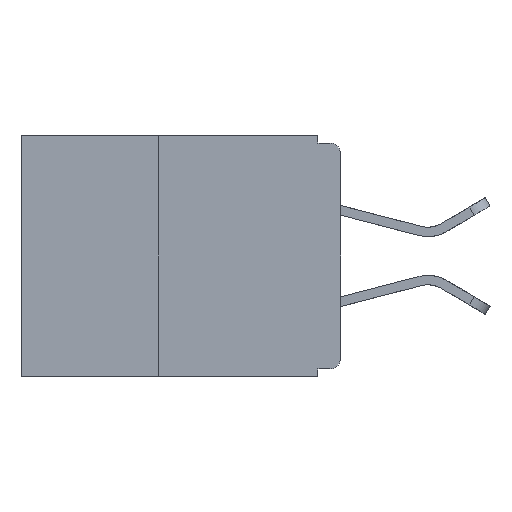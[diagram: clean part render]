
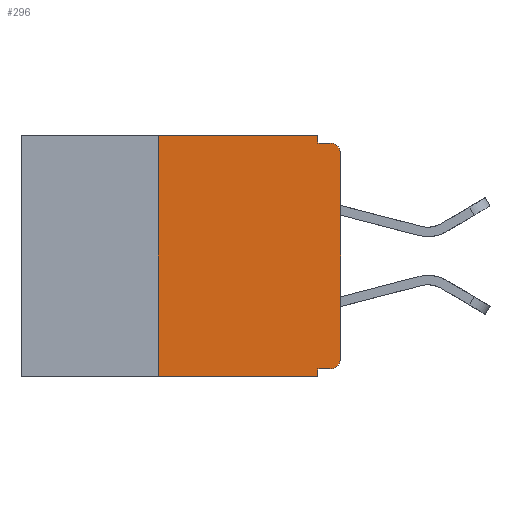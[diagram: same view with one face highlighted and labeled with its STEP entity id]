
A CAD part, left-side view. The second image highlights one B-rep face of the part: STEP entity #296.
In plain terms, the highlighted planar face has unit normal (-1, 0, 0).
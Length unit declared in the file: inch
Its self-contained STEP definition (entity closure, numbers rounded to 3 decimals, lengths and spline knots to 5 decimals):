
#296 = ADVANCED_FACE ( 'NONE', ( #11263 ), #28574, .F. ) ;
#948 = EDGE_CURVE ( 'NONE', #23775, #23313, #18565, .T. ) ;
#1109 = VERTEX_POINT ( 'NONE', #7180 ) ;
#1110 = EDGE_CURVE ( 'NONE', #29141, #15343, #18947, .T. ) ;
#1791 = CARTESIAN_POINT ( 'NONE',  ( 0., 0.25, -0.33 ) ) ;
#2021 = LINE ( 'NONE', #1791, #21980 ) ;
#2103 = CARTESIAN_POINT ( 'NONE',  ( 0., 0.031, 0. ) ) ;
#2149 = EDGE_LOOP ( 'NONE', ( #12521, #8941, #10522, #13044, #33105, #18104, #19551, #28504, #15742, #12851 ) ) ;
#2371 = VECTOR ( 'NONE', #25458, 39.37008 ) ;
#2438 = DIRECTION ( 'NONE',  ( 0., 0., -1. ) ) ;
#3979 = DIRECTION ( 'NONE',  ( 0., 0., 1. ) ) ;
#4432 = DIRECTION ( 'NONE',  ( 0., 0., 1. ) ) ;
#4693 = CARTESIAN_POINT ( 'NONE',  ( 0., 0.015, -0.01 ) ) ;
#4738 = CARTESIAN_POINT ( 'NONE',  ( 0., 0.437, 0. ) ) ;
#5278 = AXIS2_PLACEMENT_3D ( 'NONE', #27246, #6772, #20727 ) ;
#6495 = LINE ( 'NONE', #17017, #11788 ) ;
#6772 = DIRECTION ( 'NONE',  ( 1., 0., 0. ) ) ;
#7180 = CARTESIAN_POINT ( 'NONE',  ( 0., 0., -0.025 ) ) ;
#7373 = DIRECTION ( 'NONE',  ( 0., -1., 0. ) ) ;
#7431 = DIRECTION ( 'NONE',  ( -1., 0., 0. ) ) ;
#7521 = CIRCLE ( 'NONE', #15760, 0.015 ) ;
#8125 = DIRECTION ( 'NONE',  ( -1., 0., 0. ) ) ;
#8941 = ORIENTED_EDGE ( 'NONE', *, *, #21739, .T. ) ;
#10522 = ORIENTED_EDGE ( 'NONE', *, *, #11545, .F. ) ;
#11263 = FACE_OUTER_BOUND ( 'NONE', #2149, .T. ) ;
#11545 = EDGE_CURVE ( 'NONE', #23313, #26784, #32748, .T. ) ;
#11788 = VECTOR ( 'NONE', #3979, 39.37008 ) ;
#11990 = VECTOR ( 'NONE', #23617, 39.37008 ) ;
#12247 = VERTEX_POINT ( 'NONE', #26796 ) ;
#12361 = EDGE_CURVE ( 'NONE', #12247, #29141, #24601, .T. ) ;
#12521 = ORIENTED_EDGE ( 'NONE', *, *, #28033, .T. ) ;
#12851 = ORIENTED_EDGE ( 'NONE', *, *, #24973, .T. ) ;
#13044 = ORIENTED_EDGE ( 'NONE', *, *, #948, .F. ) ;
#13292 = EDGE_CURVE ( 'NONE', #14085, #23775, #30454, .T. ) ;
#13724 = CARTESIAN_POINT ( 'NONE',  ( 0., 0.031, -0.32 ) ) ;
#14085 = VERTEX_POINT ( 'NONE', #20985 ) ;
#15007 = VERTEX_POINT ( 'NONE', #32631 ) ;
#15147 = CARTESIAN_POINT ( 'NONE',  ( 0., 0.437, -0.33 ) ) ;
#15343 = VERTEX_POINT ( 'NONE', #16211 ) ;
#15742 = ORIENTED_EDGE ( 'NONE', *, *, #12361, .F. ) ;
#15760 = AXIS2_PLACEMENT_3D ( 'NONE', #23665, #8125, #26226 ) ;
#15841 = CARTESIAN_POINT ( 'NONE',  ( 0., 0.031, -0.33 ) ) ;
#16211 = CARTESIAN_POINT ( 'NONE',  ( 0., 0.031, -0.33 ) ) ;
#16932 = VECTOR ( 'NONE', #7373, 39.37008 ) ;
#17017 = CARTESIAN_POINT ( 'NONE',  ( 0., 0., 0. ) ) ;
#18104 = ORIENTED_EDGE ( 'NONE', *, *, #28184, .F. ) ;
#18565 = LINE ( 'NONE', #2103, #24544 ) ;
#18947 = LINE ( 'NONE', #15841, #11990 ) ;
#19045 = VERTEX_POINT ( 'NONE', #31705 ) ;
#19551 = ORIENTED_EDGE ( 'NONE', *, *, #28864, .T. ) ;
#20727 = DIRECTION ( 'NONE',  ( 0., 0., -1. ) ) ;
#20985 = CARTESIAN_POINT ( 'NONE',  ( 0., 0.25, 0. ) ) ;
#21359 = CIRCLE ( 'NONE', #27033, 0.015 ) ;
#21739 = EDGE_CURVE ( 'NONE', #1109, #26784, #7521, .T. ) ;
#21980 = VECTOR ( 'NONE', #4432, 39.37008 ) ;
#22987 = CARTESIAN_POINT ( 'NONE',  ( 0., 0.015, -0.305 ) ) ;
#23313 = VERTEX_POINT ( 'NONE', #30224 ) ;
#23617 = DIRECTION ( 'NONE',  ( 0., 0., -1. ) ) ;
#23665 = CARTESIAN_POINT ( 'NONE',  ( 0., 0.015, -0.025 ) ) ;
#23775 = VERTEX_POINT ( 'NONE', #31923 ) ;
#24544 = VECTOR ( 'NONE', #2438, 39.37008 ) ;
#24601 = LINE ( 'NONE', #32136, #29743 ) ;
#24973 = EDGE_CURVE ( 'NONE', #12247, #19045, #21359, .T. ) ;
#25299 = VECTOR ( 'NONE', #28945, 39.37008 ) ;
#25458 = DIRECTION ( 'NONE',  ( 0., -1., 0. ) ) ;
#25539 = DIRECTION ( 'NONE',  ( 0., 0., -1. ) ) ;
#26226 = DIRECTION ( 'NONE',  ( 0., 0., -1. ) ) ;
#26390 = CARTESIAN_POINT ( 'NONE',  ( 0., 0., -0.01 ) ) ;
#26784 = VERTEX_POINT ( 'NONE', #4693 ) ;
#26796 = CARTESIAN_POINT ( 'NONE',  ( 0., 0.015, -0.32 ) ) ;
#27033 = AXIS2_PLACEMENT_3D ( 'NONE', #22987, #7431, #25539 ) ;
#27246 = CARTESIAN_POINT ( 'NONE',  ( 0., 0.437, 0. ) ) ;
#28033 = EDGE_CURVE ( 'NONE', #19045, #1109, #6495, .T. ) ;
#28184 = EDGE_CURVE ( 'NONE', #15007, #14085, #2021, .T. ) ;
#28504 = ORIENTED_EDGE ( 'NONE', *, *, #1110, .F. ) ;
#28574 = PLANE ( 'NONE',  #5278 ) ;
#28864 = EDGE_CURVE ( 'NONE', #15007, #15343, #29894, .T. ) ;
#28945 = DIRECTION ( 'NONE',  ( 0., -1., 0. ) ) ;
#29141 = VERTEX_POINT ( 'NONE', #13724 ) ;
#29743 = VECTOR ( 'NONE', #29756, 39.37008 ) ;
#29756 = DIRECTION ( 'NONE',  ( 0., 1., 0. ) ) ;
#29894 = LINE ( 'NONE', #15147, #2371 ) ;
#30224 = CARTESIAN_POINT ( 'NONE',  ( 0., 0.031, -0.01 ) ) ;
#30454 = LINE ( 'NONE', #4738, #16932 ) ;
#31705 = CARTESIAN_POINT ( 'NONE',  ( 0., 0., -0.305 ) ) ;
#31923 = CARTESIAN_POINT ( 'NONE',  ( 0., 0.031, 0. ) ) ;
#32136 = CARTESIAN_POINT ( 'NONE',  ( 0., 0., -0.32 ) ) ;
#32631 = CARTESIAN_POINT ( 'NONE',  ( 0., 0.25, -0.33 ) ) ;
#32748 = LINE ( 'NONE', #26390, #25299 ) ;
#33105 = ORIENTED_EDGE ( 'NONE', *, *, #13292, .F. ) ;
